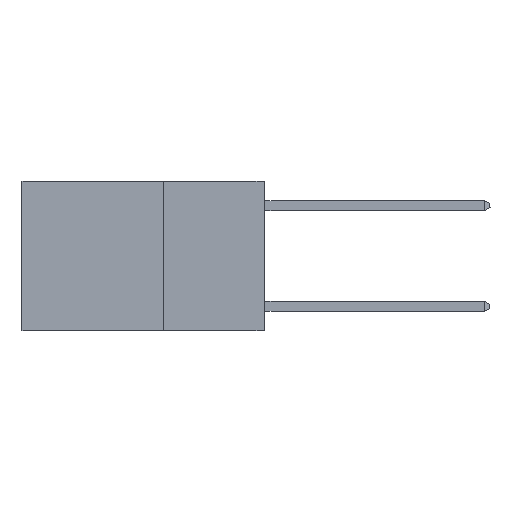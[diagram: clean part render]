
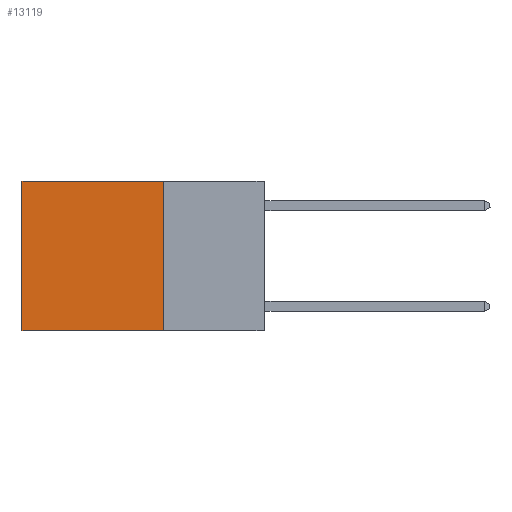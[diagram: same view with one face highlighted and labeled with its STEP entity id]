
A CAD part, left-side view. The second image highlights one B-rep face of the part: STEP entity #13119.
In plain terms, the highlighted planar face has unit normal (-1, 0, 0).
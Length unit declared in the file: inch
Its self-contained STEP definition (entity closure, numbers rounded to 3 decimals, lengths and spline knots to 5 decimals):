
#1272 = VECTOR ( 'NONE', #13260, 39.37008 ) ;
#2309 = AXIS2_PLACEMENT_3D ( 'NONE', #4979, #24060, #4732 ) ;
#3119 = DIRECTION ( 'NONE',  ( 0., 0., -1. ) ) ;
#3808 = CARTESIAN_POINT ( 'NONE',  ( 0.2625, 0.25, 0. ) ) ;
#3926 = CARTESIAN_POINT ( 'NONE',  ( 0.2625, 0.6, 0. ) ) ;
#4732 = DIRECTION ( 'NONE',  ( 0., 0., -1. ) ) ;
#4979 = CARTESIAN_POINT ( 'NONE',  ( 0.2625, 0.25, 0. ) ) ;
#6175 = ORIENTED_EDGE ( 'NONE', *, *, #9526, .T. ) ;
#6475 = LINE ( 'NONE', #3926, #1272 ) ;
#7064 = CARTESIAN_POINT ( 'NONE',  ( 0.2625, 0.25, 0. ) ) ;
#7166 = LINE ( 'NONE', #14313, #11983 ) ;
#9514 = VERTEX_POINT ( 'NONE', #7064 ) ;
#9526 = EDGE_CURVE ( 'NONE', #17732, #11052, #6475, .T. ) ;
#10008 = VECTOR ( 'NONE', #18883, 39.37008 ) ;
#11052 = VERTEX_POINT ( 'NONE', #18216 ) ;
#11288 = EDGE_CURVE ( 'NONE', #9514, #17732, #23832, .T. ) ;
#11537 = ORIENTED_EDGE ( 'NONE', *, *, #13122, .F. ) ;
#11983 = VECTOR ( 'NONE', #20912, 39.37008 ) ;
#12211 = CARTESIAN_POINT ( 'NONE',  ( 0.2625, 0.25, -0.37 ) ) ;
#13119 = ADVANCED_FACE ( 'NONE', ( #19819 ), #16238, .F. ) ;
#13122 = EDGE_CURVE ( 'NONE', #23643, #11052, #7166, .T. ) ;
#13260 = DIRECTION ( 'NONE',  ( 0., 0., -1. ) ) ;
#13735 = CARTESIAN_POINT ( 'NONE',  ( 0.2625, 0.6, 0. ) ) ;
#14313 = CARTESIAN_POINT ( 'NONE',  ( 0.2625, 0.25, -0.37 ) ) ;
#14584 = CARTESIAN_POINT ( 'NONE',  ( 0.2625, 0.25, 0. ) ) ;
#16238 = PLANE ( 'NONE',  #2309 ) ;
#17732 = VERTEX_POINT ( 'NONE', #13735 ) ;
#18216 = CARTESIAN_POINT ( 'NONE',  ( 0.2625, 0.6, -0.37 ) ) ;
#18287 = EDGE_CURVE ( 'NONE', #9514, #23643, #21058, .T. ) ;
#18680 = EDGE_LOOP ( 'NONE', ( #6175, #11537, #20095, #21044 ) ) ;
#18883 = DIRECTION ( 'NONE',  ( 0., 1., 0. ) ) ;
#19819 = FACE_OUTER_BOUND ( 'NONE', #18680, .T. ) ;
#20095 = ORIENTED_EDGE ( 'NONE', *, *, #18287, .F. ) ;
#20912 = DIRECTION ( 'NONE',  ( 0., 1., 0. ) ) ;
#21044 = ORIENTED_EDGE ( 'NONE', *, *, #11288, .T. ) ;
#21058 = LINE ( 'NONE', #14584, #22542 ) ;
#22542 = VECTOR ( 'NONE', #3119, 39.37008 ) ;
#23643 = VERTEX_POINT ( 'NONE', #12211 ) ;
#23832 = LINE ( 'NONE', #3808, #10008 ) ;
#24060 = DIRECTION ( 'NONE',  ( 1., 0., 0. ) ) ;
